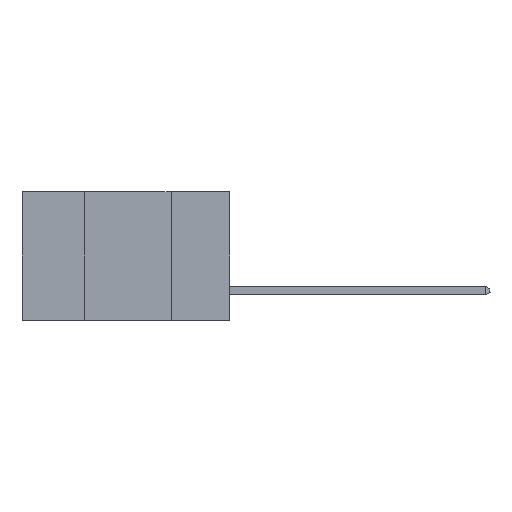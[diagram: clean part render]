
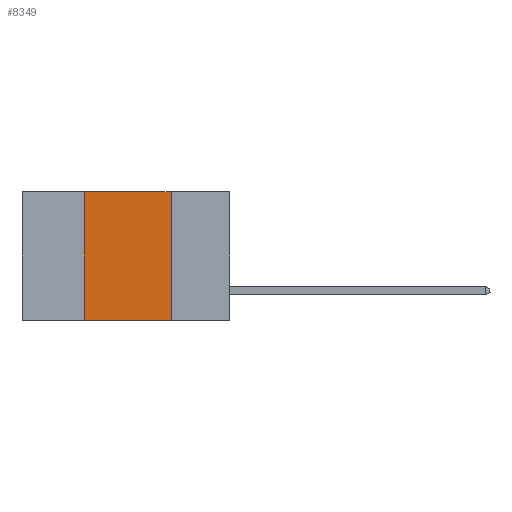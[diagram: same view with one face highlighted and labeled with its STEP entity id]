
A CAD part, left-side view. The second image highlights one B-rep face of the part: STEP entity #8349.
In plain terms, the highlighted planar face has unit normal (-1, 0, 0).
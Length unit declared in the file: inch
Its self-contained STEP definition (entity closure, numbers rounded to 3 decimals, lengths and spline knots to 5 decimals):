
#6 = DIRECTION ( 'NONE',  ( 0., -1., 0. ) ) ;
#568 = LINE ( 'NONE', #1112, #11989 ) ;
#798 = CARTESIAN_POINT ( 'NONE',  ( 0., 0.42, 0. ) ) ;
#1112 = CARTESIAN_POINT ( 'NONE',  ( 0., 0.6, 0. ) ) ;
#1264 = CARTESIAN_POINT ( 'NONE',  ( 0., 0.6, 0. ) ) ;
#2544 = VERTEX_POINT ( 'NONE', #10916 ) ;
#2722 = CARTESIAN_POINT ( 'NONE',  ( 0., 0.42, -0.37 ) ) ;
#3207 = FACE_OUTER_BOUND ( 'NONE', #7143, .T. ) ;
#3394 = LINE ( 'NONE', #798, #5657 ) ;
#3463 = DIRECTION ( 'NONE',  ( 1., 0., 0. ) ) ;
#4361 = VERTEX_POINT ( 'NONE', #10136 ) ;
#4552 = VERTEX_POINT ( 'NONE', #8794 ) ;
#5460 = VECTOR ( 'NONE', #6789, 39.37008 ) ;
#5491 = ORIENTED_EDGE ( 'NONE', *, *, #12959, .F. ) ;
#5657 = VECTOR ( 'NONE', #12378, 39.37008 ) ;
#5788 = CARTESIAN_POINT ( 'NONE',  ( 0., 0.6, -0.37 ) ) ;
#6209 = VERTEX_POINT ( 'NONE', #2722 ) ;
#6550 = VECTOR ( 'NONE', #6833, 39.37008 ) ;
#6789 = DIRECTION ( 'NONE',  ( 0., 0., -1. ) ) ;
#6833 = DIRECTION ( 'NONE',  ( 0., -1., 0. ) ) ;
#7000 = AXIS2_PLACEMENT_3D ( 'NONE', #1264, #3463, #10793 ) ;
#7143 = EDGE_LOOP ( 'NONE', ( #10709, #7615, #5491, #9249 ) ) ;
#7195 = LINE ( 'NONE', #5788, #6550 ) ;
#7615 = ORIENTED_EDGE ( 'NONE', *, *, #9961, .F. ) ;
#8349 = ADVANCED_FACE ( 'NONE', ( #3207 ), #8686, .F. ) ;
#8686 = PLANE ( 'NONE',  #7000 ) ;
#8794 = CARTESIAN_POINT ( 'NONE',  ( 0., 0.42, 0. ) ) ;
#9249 = ORIENTED_EDGE ( 'NONE', *, *, #10745, .T. ) ;
#9677 = EDGE_CURVE ( 'NONE', #4361, #2544, #11038, .T. ) ;
#9961 = EDGE_CURVE ( 'NONE', #4552, #4361, #568, .T. ) ;
#10136 = CARTESIAN_POINT ( 'NONE',  ( 0., 0.17, 0. ) ) ;
#10709 = ORIENTED_EDGE ( 'NONE', *, *, #9677, .F. ) ;
#10745 = EDGE_CURVE ( 'NONE', #6209, #2544, #7195, .T. ) ;
#10793 = DIRECTION ( 'NONE',  ( 0., 0., -1. ) ) ;
#10916 = CARTESIAN_POINT ( 'NONE',  ( 0., 0.17, -0.37 ) ) ;
#11038 = LINE ( 'NONE', #11958, #5460 ) ;
#11958 = CARTESIAN_POINT ( 'NONE',  ( 0., 0.17, 0. ) ) ;
#11989 = VECTOR ( 'NONE', #6, 39.37008 ) ;
#12378 = DIRECTION ( 'NONE',  ( 0., 0., 1. ) ) ;
#12959 = EDGE_CURVE ( 'NONE', #6209, #4552, #3394, .T. ) ;
